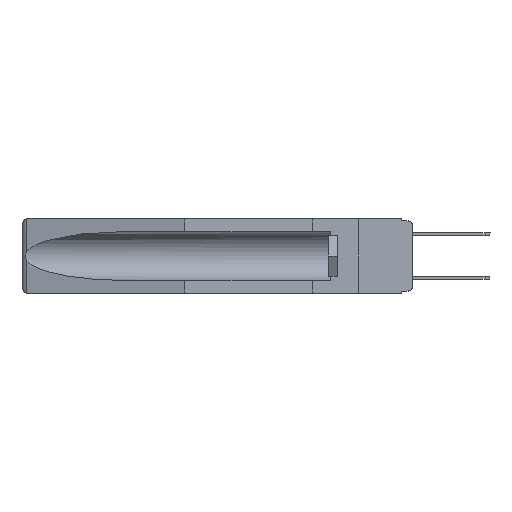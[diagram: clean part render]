
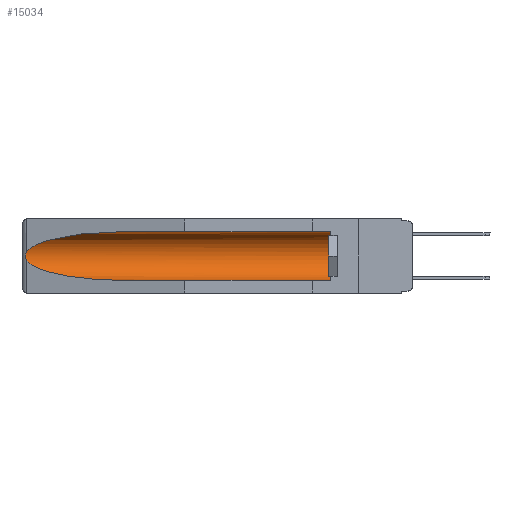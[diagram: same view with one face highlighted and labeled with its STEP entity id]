
A CAD part, left-side view. The second image highlights one B-rep face of the part: STEP entity #15034.
In plain terms, the highlighted cylindrical face has radius 2.857 mm (diameter 5.715 mm), a partial arc.
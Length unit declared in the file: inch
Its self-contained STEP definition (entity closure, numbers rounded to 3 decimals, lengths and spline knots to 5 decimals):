
#253 = CARTESIAN_POINT ( 'NONE',  ( 0.155, 1.07973, -0.284 ) ) ;
#1375 = EDGE_CURVE ( 'NONE', #18726, #21123, #6247, .T. ) ;
#1571 = CARTESIAN_POINT ( 'NONE',  ( 0.155, 0.126, -0.1715 ) ) ;
#2172 = CYLINDRICAL_SURFACE ( 'NONE', #21601, 0.1125 ) ;
#2411 = CARTESIAN_POINT ( 'NONE',  ( 0.155, 1.07973, -0.059 ) ) ;
#3185 = B_SPLINE_CURVE_WITH_KNOTS ( 'NONE', 3,
 ( #8025, #23125, #6161, #4290, #13725, #6275, #8512, #16447, #14329, #23995 ),
 .UNSPECIFIED., .F., .F.,
 ( 4, 2, 2, 2, 4 ),
 ( 0., 0.00029, 0.00058, 0.00087, 0.00117 ),
 .UNSPECIFIED. ) ;
#3634 = CARTESIAN_POINT ( 'NONE',  ( 0.155, 1.07973, -0.284 ) ) ;
#4290 = CARTESIAN_POINT ( 'NONE',  ( 0.2673, 1.5327, -0.16383 ) ) ;
#4769 = CARTESIAN_POINT ( 'NONE',  ( 0.25451, 1.48313, -0.09465 ) ) ;
#5160 = EDGE_CURVE ( 'NONE', #19019, #24265, #21033, .T. ) ;
#5969 = VERTEX_POINT ( 'NONE', #23544 ) ;
#6161 = CARTESIAN_POINT ( 'NONE',  ( 0.26654, 1.53092, -0.15636 ) ) ;
#6247 = LINE ( 'NONE', #23447, #8459 ) ;
#6275 = CARTESIAN_POINT ( 'NONE',  ( 0.2675, 1.53308, -0.17534 ) ) ;
#6383 = CARTESIAN_POINT ( 'NONE',  ( 0.26537, 1.52718, -0.14972 ) ) ;
#6726 = VECTOR ( 'NONE', #14918, 39.37008 ) ;
#7069 = CARTESIAN_POINT ( 'NONE',  ( 0.26537, 1.52718, -0.19328 ) ) ;
#8025 = CARTESIAN_POINT ( 'NONE',  ( 0.26537, 1.52718, -0.14972 ) ) ;
#8141 = CARTESIAN_POINT ( 'NONE',  ( 0.21114, 1.30732, -0.059 ) ) ;
#8442 = AXIS2_PLACEMENT_3D ( 'NONE', #1571, #24234, #12727 ) ;
#8459 = VECTOR ( 'NONE', #17640, 39.37008 ) ;
#8512 = CARTESIAN_POINT ( 'NONE',  ( 0.2673, 1.53269, -0.17917 ) ) ;
#8988 = ORIENTED_EDGE ( 'NONE', *, *, #9339, .T. ) ;
#9339 = EDGE_CURVE ( 'NONE', #10540, #18726, #10426, .T. ) ;
#9355 = CARTESIAN_POINT ( 'NONE',  ( 0.26537, 1.52718, -0.19328 ) ) ;
#9554 = CARTESIAN_POINT ( 'NONE',  ( 0.155, 0.126, -0.059 ) ) ;
#9607 = ORIENTED_EDGE ( 'NONE', *, *, #19591, .T. ) ;
#9975 = FACE_OUTER_BOUND ( 'NONE', #20023, .T. ) ;
#10426 = CIRCLE ( 'NONE', #8442, 0.1125 ) ;
#10540 = VERTEX_POINT ( 'NONE', #21299 ) ;
#11421 = ORIENTED_EDGE ( 'NONE', *, *, #5160, .T. ) ;
#11575 = ORIENTED_EDGE ( 'NONE', *, *, #1375, .T. ) ;
#12601 = ORIENTED_EDGE ( 'NONE', *, *, #14292, .T. ) ;
#12727 = DIRECTION ( 'NONE',  ( 0., 0., 1. ) ) ;
#13039 = LINE ( 'NONE', #18744, #6726 ) ;
#13708 = DIRECTION ( 'NONE',  ( 0., 1., 0. ) ) ;
#13725 = CARTESIAN_POINT ( 'NONE',  ( 0.2675, 1.53308, -0.16763 ) ) ;
#14292 = EDGE_CURVE ( 'NONE', #5969, #19019, #3185, .T. ) ;
#14329 = CARTESIAN_POINT ( 'NONE',  ( 0.26597, 1.5296, -0.19026 ) ) ;
#14918 = DIRECTION ( 'NONE',  ( 0., 1., 0. ) ) ;
#15034 = ADVANCED_FACE ( 'NONE', ( #9975 ), #2172, .F. ) ;
#15040 =( BOUNDED_CURVE ( )  B_SPLINE_CURVE ( 3, ( #2411, #8141, #4769, #6383 ),
 .UNSPECIFIED., .F., .T. ) 
 B_SPLINE_CURVE_WITH_KNOTS ( ( 4, 4 ),
 ( 4.71239, 6.08839 ),
 .UNSPECIFIED. ) 
 CURVE ( )  GEOMETRIC_REPRESENTATION_ITEM ( )  RATIONAL_B_SPLINE_CURVE ( ( 1., 0.848, 0.848, 1. ) ) 
 REPRESENTATION_ITEM ( '' )  );
#15208 = CARTESIAN_POINT ( 'NONE',  ( 0.155, -0.30754, -0.1715 ) ) ;
#16447 = CARTESIAN_POINT ( 'NONE',  ( 0.26655, 1.53094, -0.18657 ) ) ;
#16966 = ORIENTED_EDGE ( 'NONE', *, *, #21686, .F. ) ;
#17529 = DIRECTION ( 'NONE',  ( 0., 0., 1. ) ) ;
#17640 = DIRECTION ( 'NONE',  ( 0., 1., 0. ) ) ;
#18726 = VERTEX_POINT ( 'NONE', #9554 ) ;
#18744 = CARTESIAN_POINT ( 'NONE',  ( 0.155, -0.30754, -0.284 ) ) ;
#19019 = VERTEX_POINT ( 'NONE', #7069 ) ;
#19591 = EDGE_CURVE ( 'NONE', #21123, #5969, #15040, .T. ) ;
#20023 = EDGE_LOOP ( 'NONE', ( #9607, #12601, #11421, #16966, #8988, #11575 ) ) ;
#20141 = CARTESIAN_POINT ( 'NONE',  ( 0.155, 1.07973, -0.059 ) ) ;
#20620 = CARTESIAN_POINT ( 'NONE',  ( 0.25451, 1.48313, -0.24835 ) ) ;
#21033 =( BOUNDED_CURVE ( )  B_SPLINE_CURVE ( 3, ( #9355, #20620, #22592, #3634 ),
 .UNSPECIFIED., .F., .T. ) 
 B_SPLINE_CURVE_WITH_KNOTS ( ( 4, 4 ),
 ( 0.1948, 1.5708 ),
 .UNSPECIFIED. ) 
 CURVE ( )  GEOMETRIC_REPRESENTATION_ITEM ( )  RATIONAL_B_SPLINE_CURVE ( ( 1., 0.848, 0.848, 1. ) ) 
 REPRESENTATION_ITEM ( '' )  );
#21123 = VERTEX_POINT ( 'NONE', #20141 ) ;
#21299 = CARTESIAN_POINT ( 'NONE',  ( 0.155, 0.126, -0.284 ) ) ;
#21601 = AXIS2_PLACEMENT_3D ( 'NONE', #15208, #13708, #17529 ) ;
#21686 = EDGE_CURVE ( 'NONE', #10540, #24265, #13039, .T. ) ;
#22592 = CARTESIAN_POINT ( 'NONE',  ( 0.21114, 1.30732, -0.284 ) ) ;
#23125 = CARTESIAN_POINT ( 'NONE',  ( 0.26597, 1.52961, -0.15275 ) ) ;
#23447 = CARTESIAN_POINT ( 'NONE',  ( 0.155, -0.30754, -0.059 ) ) ;
#23544 = CARTESIAN_POINT ( 'NONE',  ( 0.26537, 1.52718, -0.14972 ) ) ;
#23995 = CARTESIAN_POINT ( 'NONE',  ( 0.26537, 1.52718, -0.19328 ) ) ;
#24234 = DIRECTION ( 'NONE',  ( 0., -1., 0. ) ) ;
#24265 = VERTEX_POINT ( 'NONE', #253 ) ;
